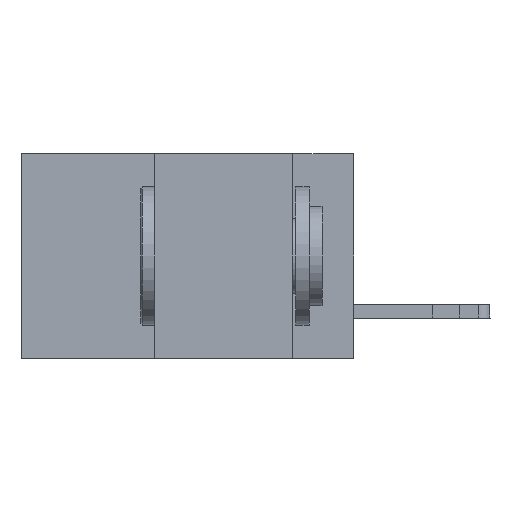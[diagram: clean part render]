
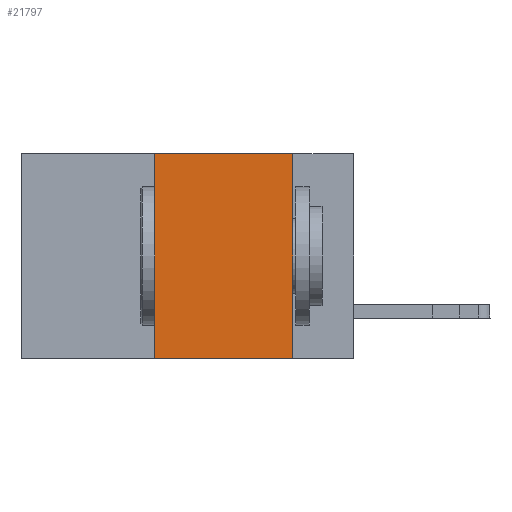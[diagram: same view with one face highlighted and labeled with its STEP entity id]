
A CAD part, left-side view. The second image highlights one B-rep face of the part: STEP entity #21797.
In plain terms, the highlighted planar face has unit normal (-1, 0, 0).
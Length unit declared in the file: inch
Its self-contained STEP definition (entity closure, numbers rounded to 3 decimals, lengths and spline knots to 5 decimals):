
#31 = EDGE_CURVE ( 'NONE', #21209, #34669, #2418, .T. ) ;
#207 = DIRECTION ( 'NONE',  ( 1., 0., 0. ) ) ;
#710 = VECTOR ( 'NONE', #25065, 39.37008 ) ;
#1474 = ORIENTED_EDGE ( 'NONE', *, *, #31746, .F. ) ;
#2418 = LINE ( 'NONE', #10929, #710 ) ;
#4164 = EDGE_CURVE ( 'NONE', #27502, #32163, #15352, .T. ) ;
#4561 = DIRECTION ( 'NONE',  ( 0., -1., 0. ) ) ;
#5272 = CARTESIAN_POINT ( 'NONE',  ( 0., 0.11, -0.37 ) ) ;
#5936 = DIRECTION ( 'NONE',  ( 0., 0., -1. ) ) ;
#6894 = VECTOR ( 'NONE', #18809, 39.37008 ) ;
#7224 = EDGE_CURVE ( 'NONE', #27502, #34669, #29807, .T. ) ;
#7561 = ORIENTED_EDGE ( 'NONE', *, *, #4164, .F. ) ;
#10388 = EDGE_LOOP ( 'NONE', ( #15957, #1474, #7561, #10594 ) ) ;
#10594 = ORIENTED_EDGE ( 'NONE', *, *, #7224, .T. ) ;
#10929 = CARTESIAN_POINT ( 'NONE',  ( 0., 0.11, 0. ) ) ;
#12313 = LINE ( 'NONE', #34936, #6894 ) ;
#12712 = CARTESIAN_POINT ( 'NONE',  ( 0., 0.6, -0.37 ) ) ;
#15352 = LINE ( 'NONE', #18340, #16686 ) ;
#15683 = CARTESIAN_POINT ( 'NONE',  ( 0., 0.36, 0. ) ) ;
#15957 = ORIENTED_EDGE ( 'NONE', *, *, #31, .F. ) ;
#16686 = VECTOR ( 'NONE', #26724, 39.37008 ) ;
#17476 = VECTOR ( 'NONE', #4561, 39.37008 ) ;
#18340 = CARTESIAN_POINT ( 'NONE',  ( 0., 0.36, 0. ) ) ;
#18809 = DIRECTION ( 'NONE',  ( 0., -1., 0. ) ) ;
#20057 = FACE_OUTER_BOUND ( 'NONE', #10388, .T. ) ;
#21209 = VERTEX_POINT ( 'NONE', #23712 ) ;
#21797 = ADVANCED_FACE ( 'NONE', ( #20057 ), #28448, .F. ) ;
#22530 = AXIS2_PLACEMENT_3D ( 'NONE', #25641, #207, #5936 ) ;
#23198 = CARTESIAN_POINT ( 'NONE',  ( 0., 0.36, -0.37 ) ) ;
#23712 = CARTESIAN_POINT ( 'NONE',  ( 0., 0.11, 0. ) ) ;
#25065 = DIRECTION ( 'NONE',  ( 0., 0., -1. ) ) ;
#25641 = CARTESIAN_POINT ( 'NONE',  ( 0., 0.6, 0. ) ) ;
#26724 = DIRECTION ( 'NONE',  ( 0., 0., 1. ) ) ;
#27502 = VERTEX_POINT ( 'NONE', #23198 ) ;
#28448 = PLANE ( 'NONE',  #22530 ) ;
#29807 = LINE ( 'NONE', #12712, #17476 ) ;
#31746 = EDGE_CURVE ( 'NONE', #32163, #21209, #12313, .T. ) ;
#32163 = VERTEX_POINT ( 'NONE', #15683 ) ;
#34669 = VERTEX_POINT ( 'NONE', #5272 ) ;
#34936 = CARTESIAN_POINT ( 'NONE',  ( 0., 0.6, 0. ) ) ;
